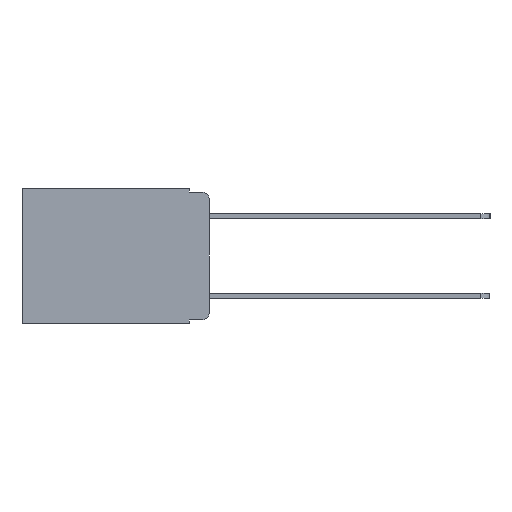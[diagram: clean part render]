
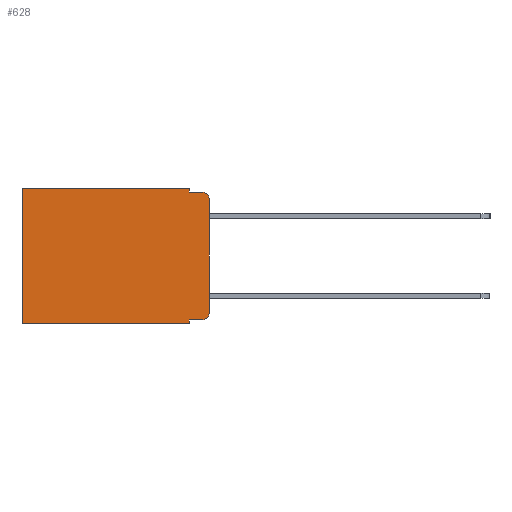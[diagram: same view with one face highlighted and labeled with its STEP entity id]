
A CAD part, left-side view. The second image highlights one B-rep face of the part: STEP entity #628.
In plain terms, the highlighted planar face has unit normal (-1, 0, 0).
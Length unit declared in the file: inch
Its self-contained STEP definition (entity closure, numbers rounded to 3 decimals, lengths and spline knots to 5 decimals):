
#107 = VECTOR ( 'NONE', #7031, 39.37008 ) ;
#189 = CARTESIAN_POINT ( 'NONE',  ( 0.298, 0.051, -0.01 ) ) ;
#373 = VERTEX_POINT ( 'NONE', #12287 ) ;
#534 = LINE ( 'NONE', #9143, #3900 ) ;
#628 = ADVANCED_FACE ( 'NONE', ( #5924 ), #1028, .F. ) ;
#1028 = PLANE ( 'NONE',  #1813 ) ;
#1181 = CARTESIAN_POINT ( 'NONE',  ( 0.298, 0.02, -0.313 ) ) ;
#1355 = DIRECTION ( 'NONE',  ( 0., 0., -1. ) ) ;
#1366 = DIRECTION ( 'NONE',  ( 1., 0., 0. ) ) ;
#1606 = DIRECTION ( 'NONE',  ( 0., 0., -1. ) ) ;
#1813 = AXIS2_PLACEMENT_3D ( 'NONE', #15947, #1366, #1355 ) ;
#2583 = ORIENTED_EDGE ( 'NONE', *, *, #17212, .F. ) ;
#2901 = DIRECTION ( 'NONE',  ( 0., 0., -1. ) ) ;
#3085 = EDGE_CURVE ( 'NONE', #3343, #373, #534, .T. ) ;
#3226 = VERTEX_POINT ( 'NONE', #7403 ) ;
#3343 = VERTEX_POINT ( 'NONE', #16031 ) ;
#3432 = DIRECTION ( 'NONE',  ( 0., -1., 0. ) ) ;
#3644 = EDGE_CURVE ( 'NONE', #3226, #373, #19315, .T. ) ;
#3900 = VECTOR ( 'NONE', #14310, 39.37008 ) ;
#4328 = ORIENTED_EDGE ( 'NONE', *, *, #19086, .F. ) ;
#4715 = LINE ( 'NONE', #16323, #16309 ) ;
#4748 = EDGE_CURVE ( 'NONE', #17777, #16038, #13567, .T. ) ;
#4837 = ORIENTED_EDGE ( 'NONE', *, *, #3644, .T. ) ;
#4930 = EDGE_CURVE ( 'NONE', #12159, #3226, #14662, .T. ) ;
#5039 = CIRCLE ( 'NONE', #13285, 0.02 ) ;
#5072 = CARTESIAN_POINT ( 'NONE',  ( 0.298, 0., 0. ) ) ;
#5486 = VECTOR ( 'NONE', #1606, 39.37008 ) ;
#5501 = EDGE_LOOP ( 'NONE', ( #14217, #19247, #19681, #4328, #16425, #4837, #5813, #2583, #11947, #16940 ) ) ;
#5567 = CARTESIAN_POINT ( 'NONE',  ( 0.298, 0.051, 0. ) ) ;
#5813 = ORIENTED_EDGE ( 'NONE', *, *, #3085, .F. ) ;
#5822 = VECTOR ( 'NONE', #14574, 39.37008 ) ;
#5924 = FACE_OUTER_BOUND ( 'NONE', #5501, .T. ) ;
#6257 = CARTESIAN_POINT ( 'NONE',  ( 0.298, 0.02, -0.03 ) ) ;
#7031 = DIRECTION ( 'NONE',  ( 0., 0., -1. ) ) ;
#7165 = CARTESIAN_POINT ( 'NONE',  ( 0.298, 0.051, -0.333 ) ) ;
#7256 = VERTEX_POINT ( 'NONE', #11461 ) ;
#7403 = CARTESIAN_POINT ( 'NONE',  ( 0.298, 0.473, 0. ) ) ;
#7858 = VERTEX_POINT ( 'NONE', #19454 ) ;
#7866 = DIRECTION ( 'NONE',  ( 0., 0., -1. ) ) ;
#7903 = EDGE_CURVE ( 'NONE', #7256, #16038, #9185, .T. ) ;
#8161 = CARTESIAN_POINT ( 'NONE',  ( 0.298, 0.051, -0.333 ) ) ;
#8797 = LINE ( 'NONE', #5567, #107 ) ;
#8973 = DIRECTION ( 'NONE',  ( 0., 0., -1. ) ) ;
#8996 = EDGE_CURVE ( 'NONE', #7256, #13566, #4715, .T. ) ;
#9143 = CARTESIAN_POINT ( 'NONE',  ( 0.298, 0., -0.343 ) ) ;
#9185 = CIRCLE ( 'NONE', #11156, 0.02 ) ;
#9384 = CARTESIAN_POINT ( 'NONE',  ( 0.298, 0.473, 0. ) ) ;
#10436 = CARTESIAN_POINT ( 'NONE',  ( 0.298, 0., -0.313 ) ) ;
#11137 = CARTESIAN_POINT ( 'NONE',  ( 0.298, 0.051, 0. ) ) ;
#11156 = AXIS2_PLACEMENT_3D ( 'NONE', #6257, #16772, #7866 ) ;
#11440 = EDGE_CURVE ( 'NONE', #17267, #7858, #17295, .T. ) ;
#11461 = CARTESIAN_POINT ( 'NONE',  ( 0.298, 0., -0.03 ) ) ;
#11947 = ORIENTED_EDGE ( 'NONE', *, *, #11440, .T. ) ;
#12159 = VERTEX_POINT ( 'NONE', #13306 ) ;
#12287 = CARTESIAN_POINT ( 'NONE',  ( 0.298, 0.473, -0.343 ) ) ;
#12307 = DIRECTION ( 'NONE',  ( -1., 0., 0. ) ) ;
#12804 = LINE ( 'NONE', #11137, #5486 ) ;
#13285 = AXIS2_PLACEMENT_3D ( 'NONE', #1181, #12307, #2901 ) ;
#13306 = CARTESIAN_POINT ( 'NONE',  ( 0.298, 0.051, 0. ) ) ;
#13566 = VERTEX_POINT ( 'NONE', #10436 ) ;
#13567 = LINE ( 'NONE', #17382, #5822 ) ;
#14217 = ORIENTED_EDGE ( 'NONE', *, *, #8996, .F. ) ;
#14310 = DIRECTION ( 'NONE',  ( 0., 1., 0. ) ) ;
#14574 = DIRECTION ( 'NONE',  ( 0., -1., 0. ) ) ;
#14662 = LINE ( 'NONE', #5072, #17933 ) ;
#15947 = CARTESIAN_POINT ( 'NONE',  ( 0.298, 0., 0. ) ) ;
#16031 = CARTESIAN_POINT ( 'NONE',  ( 0.298, 0.051, -0.343 ) ) ;
#16038 = VERTEX_POINT ( 'NONE', #19076 ) ;
#16309 = VECTOR ( 'NONE', #8973, 39.37008 ) ;
#16317 = DIRECTION ( 'NONE',  ( 0., 0., -1. ) ) ;
#16323 = CARTESIAN_POINT ( 'NONE',  ( 0.298, 0., 0. ) ) ;
#16425 = ORIENTED_EDGE ( 'NONE', *, *, #4930, .T. ) ;
#16772 = DIRECTION ( 'NONE',  ( -1., 0., 0. ) ) ;
#16866 = VECTOR ( 'NONE', #3432, 39.37008 ) ;
#16940 = ORIENTED_EDGE ( 'NONE', *, *, #18127, .T. ) ;
#17212 = EDGE_CURVE ( 'NONE', #17267, #3343, #8797, .T. ) ;
#17267 = VERTEX_POINT ( 'NONE', #7165 ) ;
#17295 = LINE ( 'NONE', #8161, #16866 ) ;
#17382 = CARTESIAN_POINT ( 'NONE',  ( 0.298, 0.051, -0.01 ) ) ;
#17777 = VERTEX_POINT ( 'NONE', #189 ) ;
#17933 = VECTOR ( 'NONE', #18420, 39.37008 ) ;
#18127 = EDGE_CURVE ( 'NONE', #7858, #13566, #5039, .T. ) ;
#18420 = DIRECTION ( 'NONE',  ( 0., 1., 0. ) ) ;
#18877 = VECTOR ( 'NONE', #16317, 39.37008 ) ;
#19076 = CARTESIAN_POINT ( 'NONE',  ( 0.298, 0.02, -0.01 ) ) ;
#19086 = EDGE_CURVE ( 'NONE', #12159, #17777, #12804, .T. ) ;
#19247 = ORIENTED_EDGE ( 'NONE', *, *, #7903, .T. ) ;
#19315 = LINE ( 'NONE', #9384, #18877 ) ;
#19454 = CARTESIAN_POINT ( 'NONE',  ( 0.298, 0.02, -0.333 ) ) ;
#19681 = ORIENTED_EDGE ( 'NONE', *, *, #4748, .F. ) ;
